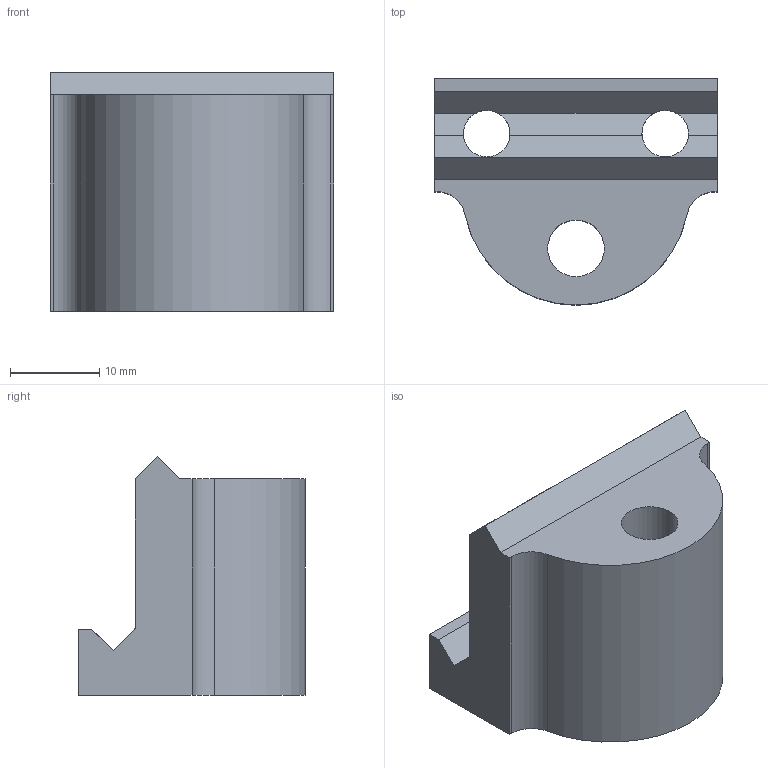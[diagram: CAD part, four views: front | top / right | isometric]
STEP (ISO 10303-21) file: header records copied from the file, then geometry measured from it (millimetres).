
FILE_DESCRIPTION(/* description */ ('STEP AP214'),/* implementation_level */ '2;1');
FILE_NAME(/* name */ 'Mount.stp',/* time_stamp */ '2019-08-10T22:58:26-05:00',/* author */ ('johne'),/* organization */ (''),/* preprocessor_version */ 'ST-DEVELOPER v16.13',/* originating_system */ 'Autodesk Inventor 2018',/* authorisation */ '');
FILE_SCHEMA (('AUTOMOTIVE_DESIGN { 1 0 10303 214 3 1 1 }'));
Length unit declared in the file: inch
Products named in the file (1): Mount
Bounding box: 31.75 x 25.4 x 26.75 mm (x, y, z)
Volume: 11202 mm3; surface area: 4327.4 mm2
Topology: 1 solids, 1 shells, 25 faces, 73 edges, 48 vertices
Faces by surface type: plane 17, cylinder 6, cone 2
Full cylindrical faces by diameter (mm): 5.232 x2, 6.35 x1
Entity records: 841 total; most frequent: DIRECTION 138, CARTESIAN_POINT 138, ORIENTED_EDGE 132, EDGE_CURVE 66, LINE 46, VECTOR 46, VERTEX_POINT 46, AXIS2_PLACEMENT_3D 46
